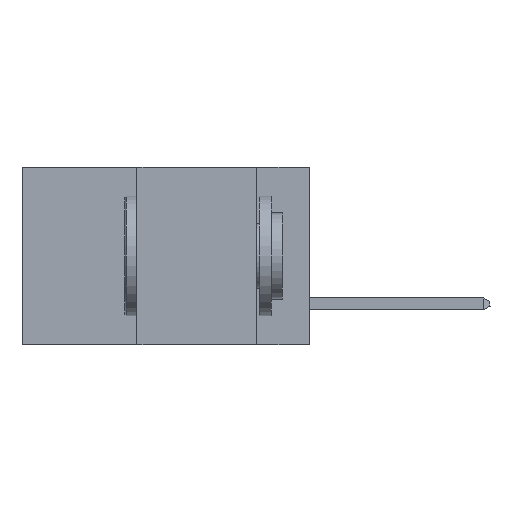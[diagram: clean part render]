
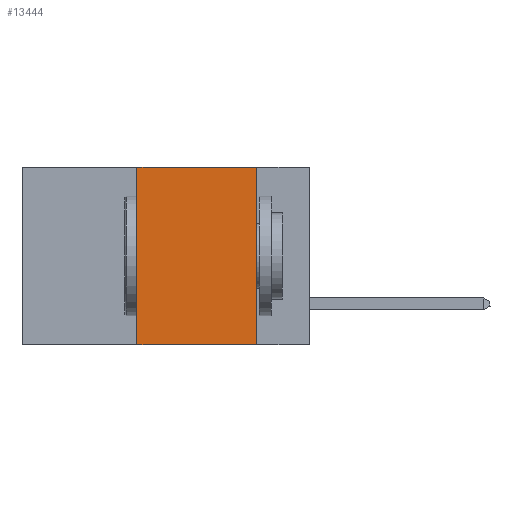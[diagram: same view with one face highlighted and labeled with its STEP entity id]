
A CAD part, left-side view. The second image highlights one B-rep face of the part: STEP entity #13444.
In plain terms, the highlighted planar face has unit normal (-1, 0, 0).
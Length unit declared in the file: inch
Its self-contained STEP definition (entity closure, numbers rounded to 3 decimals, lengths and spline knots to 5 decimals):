
#187 = VECTOR ( 'NONE', #462, 39.37008 ) ;
#462 = DIRECTION ( 'NONE',  ( 0., -1., 0. ) ) ;
#865 = CARTESIAN_POINT ( 'NONE',  ( 0., 0.11, 0. ) ) ;
#1328 = CARTESIAN_POINT ( 'NONE',  ( 0., 0.6, -0.37 ) ) ;
#1529 = VERTEX_POINT ( 'NONE', #6243 ) ;
#3289 = EDGE_CURVE ( 'NONE', #9322, #8645, #11167, .T. ) ;
#3699 = LINE ( 'NONE', #1328, #187 ) ;
#3964 = ORIENTED_EDGE ( 'NONE', *, *, #8838, .F. ) ;
#3979 = AXIS2_PLACEMENT_3D ( 'NONE', #5167, #12667, #10438 ) ;
#5167 = CARTESIAN_POINT ( 'NONE',  ( 0., 0.6, 0. ) ) ;
#5297 = VECTOR ( 'NONE', #7346, 39.37008 ) ;
#5969 = FACE_OUTER_BOUND ( 'NONE', #12994, .T. ) ;
#6243 = CARTESIAN_POINT ( 'NONE',  ( 0., 0.11, 0. ) ) ;
#6433 = CARTESIAN_POINT ( 'NONE',  ( 0., 0.6, 0. ) ) ;
#6899 = VECTOR ( 'NONE', #8283, 39.37008 ) ;
#7346 = DIRECTION ( 'NONE',  ( 0., 0., 1. ) ) ;
#7538 = VERTEX_POINT ( 'NONE', #9032 ) ;
#7683 = ORIENTED_EDGE ( 'NONE', *, *, #3289, .F. ) ;
#8182 = DIRECTION ( 'NONE',  ( 0., -1., 0. ) ) ;
#8283 = DIRECTION ( 'NONE',  ( 0., 0., -1. ) ) ;
#8633 = ORIENTED_EDGE ( 'NONE', *, *, #11941, .T. ) ;
#8645 = VERTEX_POINT ( 'NONE', #11214 ) ;
#8838 = EDGE_CURVE ( 'NONE', #8645, #1529, #13262, .T. ) ;
#8896 = EDGE_CURVE ( 'NONE', #1529, #7538, #9770, .T. ) ;
#9032 = CARTESIAN_POINT ( 'NONE',  ( 0., 0.11, -0.37 ) ) ;
#9322 = VERTEX_POINT ( 'NONE', #11832 ) ;
#9770 = LINE ( 'NONE', #865, #6899 ) ;
#10434 = VECTOR ( 'NONE', #8182, 39.37008 ) ;
#10438 = DIRECTION ( 'NONE',  ( 0., 0., -1. ) ) ;
#10560 = ORIENTED_EDGE ( 'NONE', *, *, #8896, .F. ) ;
#11167 = LINE ( 'NONE', #13779, #5297 ) ;
#11214 = CARTESIAN_POINT ( 'NONE',  ( 0., 0.36, 0. ) ) ;
#11584 = PLANE ( 'NONE',  #3979 ) ;
#11832 = CARTESIAN_POINT ( 'NONE',  ( 0., 0.36, -0.37 ) ) ;
#11941 = EDGE_CURVE ( 'NONE', #9322, #7538, #3699, .T. ) ;
#12667 = DIRECTION ( 'NONE',  ( 1., 0., 0. ) ) ;
#12994 = EDGE_LOOP ( 'NONE', ( #10560, #3964, #7683, #8633 ) ) ;
#13262 = LINE ( 'NONE', #6433, #10434 ) ;
#13444 = ADVANCED_FACE ( 'NONE', ( #5969 ), #11584, .F. ) ;
#13779 = CARTESIAN_POINT ( 'NONE',  ( 0., 0.36, 0. ) ) ;
